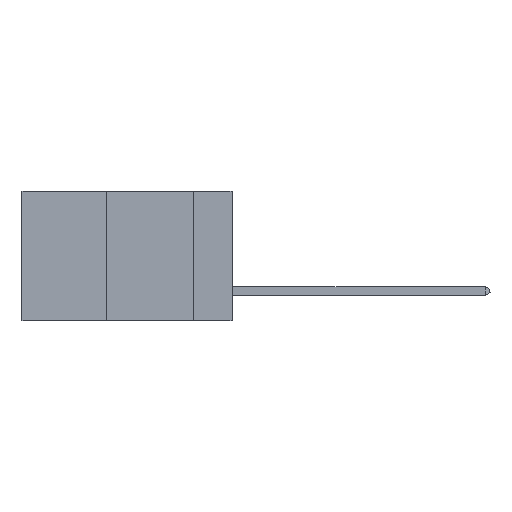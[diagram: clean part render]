
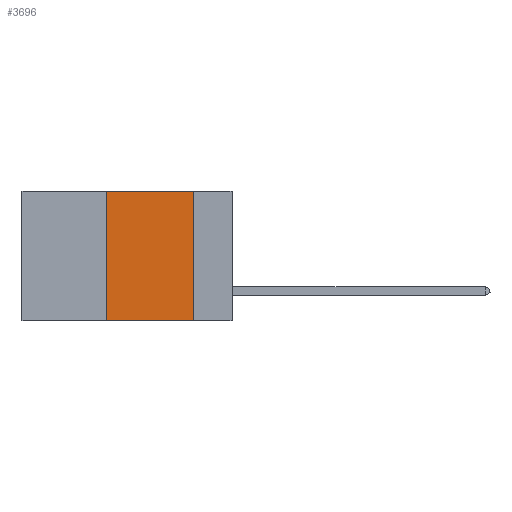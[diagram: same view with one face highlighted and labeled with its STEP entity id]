
A CAD part, left-side view. The second image highlights one B-rep face of the part: STEP entity #3696.
In plain terms, the highlighted planar face has unit normal (-1, 0, 0).
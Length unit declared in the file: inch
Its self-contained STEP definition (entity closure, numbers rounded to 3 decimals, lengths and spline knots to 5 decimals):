
#321 = EDGE_CURVE ( 'NONE', #967, #1288, #9521, .T. ) ;
#960 = ORIENTED_EDGE ( 'NONE', *, *, #321, .F. ) ;
#967 = VERTEX_POINT ( 'NONE', #8211 ) ;
#1083 = VECTOR ( 'NONE', #1970, 39.37008 ) ;
#1288 = VERTEX_POINT ( 'NONE', #7252 ) ;
#1327 = AXIS2_PLACEMENT_3D ( 'NONE', #3019, #7879, #5800 ) ;
#1532 = EDGE_LOOP ( 'NONE', ( #10772, #11911, #960, #5091 ) ) ;
#1970 = DIRECTION ( 'NONE',  ( 0., 0., -1. ) ) ;
#2120 = LINE ( 'NONE', #11370, #8601 ) ;
#2886 = VECTOR ( 'NONE', #3597, 39.37008 ) ;
#3019 = CARTESIAN_POINT ( 'NONE',  ( 0., 0.6, 0. ) ) ;
#3244 = FACE_OUTER_BOUND ( 'NONE', #1532, .T. ) ;
#3597 = DIRECTION ( 'NONE',  ( 0., 0., 1. ) ) ;
#3696 = ADVANCED_FACE ( 'NONE', ( #3244 ), #6931, .F. ) ;
#3847 = DIRECTION ( 'NONE',  ( 0., -1., 0. ) ) ;
#3874 = CARTESIAN_POINT ( 'NONE',  ( 0., 0.11, -0.37 ) ) ;
#4125 = LINE ( 'NONE', #9576, #11941 ) ;
#5091 = ORIENTED_EDGE ( 'NONE', *, *, #5278, .T. ) ;
#5278 = EDGE_CURVE ( 'NONE', #967, #12409, #4125, .T. ) ;
#5681 = DIRECTION ( 'NONE',  ( 0., -1., 0. ) ) ;
#5800 = DIRECTION ( 'NONE',  ( 0., 0., -1. ) ) ;
#6457 = CARTESIAN_POINT ( 'NONE',  ( 0., 0.36, 0. ) ) ;
#6478 = VERTEX_POINT ( 'NONE', #11754 ) ;
#6931 = PLANE ( 'NONE',  #1327 ) ;
#7073 = LINE ( 'NONE', #7722, #1083 ) ;
#7252 = CARTESIAN_POINT ( 'NONE',  ( 0., 0.36, 0. ) ) ;
#7722 = CARTESIAN_POINT ( 'NONE',  ( 0., 0.11, 0. ) ) ;
#7879 = DIRECTION ( 'NONE',  ( 1., 0., 0. ) ) ;
#8211 = CARTESIAN_POINT ( 'NONE',  ( 0., 0.36, -0.37 ) ) ;
#8601 = VECTOR ( 'NONE', #5681, 39.37008 ) ;
#8967 = EDGE_CURVE ( 'NONE', #1288, #6478, #2120, .T. ) ;
#9521 = LINE ( 'NONE', #6457, #2886 ) ;
#9576 = CARTESIAN_POINT ( 'NONE',  ( 0., 0.6, -0.37 ) ) ;
#10326 = EDGE_CURVE ( 'NONE', #6478, #12409, #7073, .T. ) ;
#10772 = ORIENTED_EDGE ( 'NONE', *, *, #10326, .F. ) ;
#11370 = CARTESIAN_POINT ( 'NONE',  ( 0., 0.6, 0. ) ) ;
#11754 = CARTESIAN_POINT ( 'NONE',  ( 0., 0.11, 0. ) ) ;
#11911 = ORIENTED_EDGE ( 'NONE', *, *, #8967, .F. ) ;
#11941 = VECTOR ( 'NONE', #3847, 39.37008 ) ;
#12409 = VERTEX_POINT ( 'NONE', #3874 ) ;
